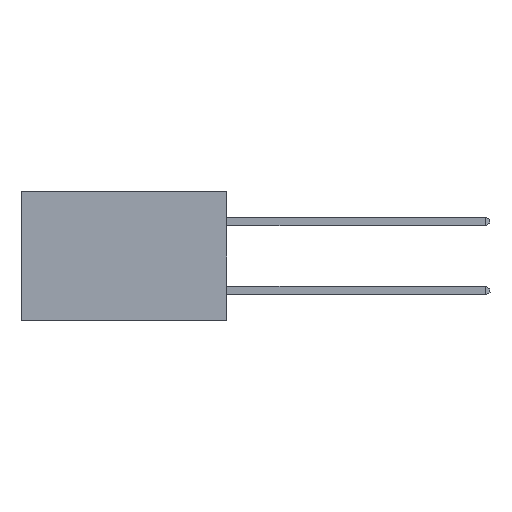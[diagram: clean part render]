
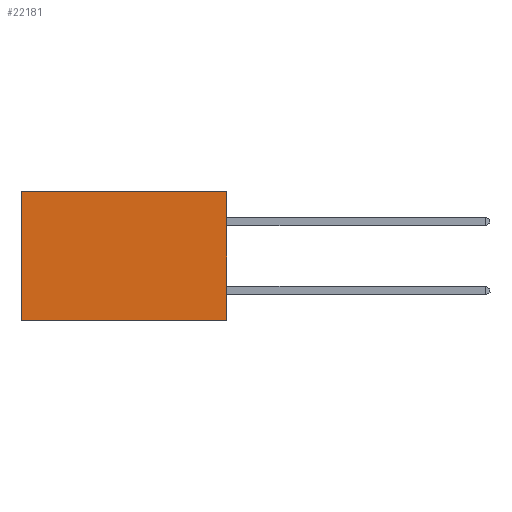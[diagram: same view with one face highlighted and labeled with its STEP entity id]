
A CAD part, left-side view. The second image highlights one B-rep face of the part: STEP entity #22181.
In plain terms, the highlighted planar face has unit normal (-1, 0, 0).
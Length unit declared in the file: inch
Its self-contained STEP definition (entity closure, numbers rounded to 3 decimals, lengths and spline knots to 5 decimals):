
#1122 = LINE ( 'NONE', #9333, #9258 ) ;
#2493 = VERTEX_POINT ( 'NONE', #9512 ) ;
#3145 = CARTESIAN_POINT ( 'NONE',  ( 0.277, 0.59, -0.37 ) ) ;
#3254 = FACE_OUTER_BOUND ( 'NONE', #15498, .T. ) ;
#3832 = ORIENTED_EDGE ( 'NONE', *, *, #4554, .T. ) ;
#3974 = LINE ( 'NONE', #18711, #20224 ) ;
#4085 = LINE ( 'NONE', #3145, #16931 ) ;
#4139 = DIRECTION ( 'NONE',  ( 0., 1., 0. ) ) ;
#4326 = EDGE_CURVE ( 'NONE', #13294, #2493, #12387, .T. ) ;
#4554 = EDGE_CURVE ( 'NONE', #13294, #15234, #3974, .T. ) ;
#5984 = DIRECTION ( 'NONE',  ( 0., 0., -1. ) ) ;
#6275 = CARTESIAN_POINT ( 'NONE',  ( 0.277, 0., -0.37 ) ) ;
#7353 = CARTESIAN_POINT ( 'NONE',  ( 0.277, 0., -0.37 ) ) ;
#8357 = CARTESIAN_POINT ( 'NONE',  ( 0.277, 0.59, -0.37 ) ) ;
#9103 = DIRECTION ( 'NONE',  ( 1., 0., 0. ) ) ;
#9258 = VECTOR ( 'NONE', #4139, 39.37008 ) ;
#9333 = CARTESIAN_POINT ( 'NONE',  ( 0.277, 0., -0.37 ) ) ;
#9512 = CARTESIAN_POINT ( 'NONE',  ( 0.277, 0., -0.37 ) ) ;
#10094 = AXIS2_PLACEMENT_3D ( 'NONE', #7353, #9103, #21171 ) ;
#12244 = ORIENTED_EDGE ( 'NONE', *, *, #17727, .T. ) ;
#12387 = LINE ( 'NONE', #6275, #12938 ) ;
#12938 = VECTOR ( 'NONE', #5984, 39.37008 ) ;
#13294 = VERTEX_POINT ( 'NONE', #15927 ) ;
#15234 = VERTEX_POINT ( 'NONE', #19839 ) ;
#15498 = EDGE_LOOP ( 'NONE', ( #12244, #17551, #20559, #3832 ) ) ;
#15927 = CARTESIAN_POINT ( 'NONE',  ( 0.277, 0., 0. ) ) ;
#16235 = VERTEX_POINT ( 'NONE', #8357 ) ;
#16931 = VECTOR ( 'NONE', #22141, 39.37008 ) ;
#17551 = ORIENTED_EDGE ( 'NONE', *, *, #18129, .F. ) ;
#17727 = EDGE_CURVE ( 'NONE', #15234, #16235, #4085, .T. ) ;
#17795 = PLANE ( 'NONE',  #10094 ) ;
#18129 = EDGE_CURVE ( 'NONE', #2493, #16235, #1122, .T. ) ;
#18711 = CARTESIAN_POINT ( 'NONE',  ( 0.277, 0., 0. ) ) ;
#19839 = CARTESIAN_POINT ( 'NONE',  ( 0.277, 0.59, 0. ) ) ;
#20224 = VECTOR ( 'NONE', #20648, 39.37008 ) ;
#20559 = ORIENTED_EDGE ( 'NONE', *, *, #4326, .F. ) ;
#20648 = DIRECTION ( 'NONE',  ( 0., 1., 0. ) ) ;
#21171 = DIRECTION ( 'NONE',  ( 0., 0., -1. ) ) ;
#22141 = DIRECTION ( 'NONE',  ( 0., 0., -1. ) ) ;
#22181 = ADVANCED_FACE ( 'NONE', ( #3254 ), #17795, .F. ) ;
